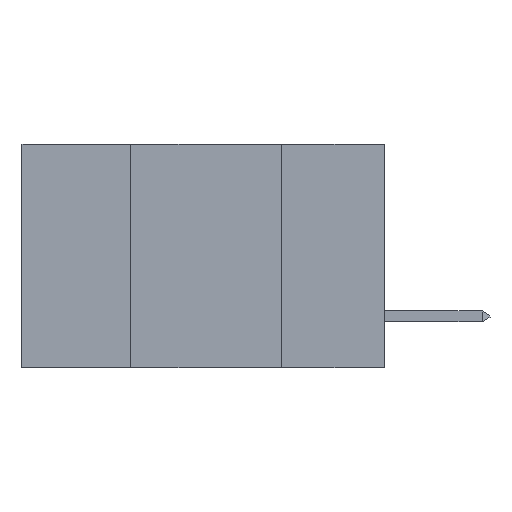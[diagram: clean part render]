
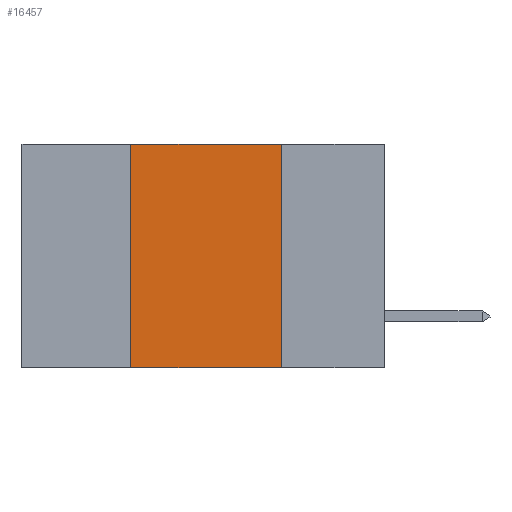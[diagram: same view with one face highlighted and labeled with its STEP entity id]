
A CAD part, left-side view. The second image highlights one B-rep face of the part: STEP entity #16457.
In plain terms, the highlighted planar face has unit normal (-1, 0, 0).
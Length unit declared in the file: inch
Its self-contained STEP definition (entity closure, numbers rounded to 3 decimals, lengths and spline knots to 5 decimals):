
#475 = CARTESIAN_POINT ( 'NONE',  ( 0., 0.17, 0. ) ) ;
#1686 = EDGE_CURVE ( 'NONE', #9627, #5954, #11650, .T. ) ;
#2778 = DIRECTION ( 'NONE',  ( 0., -1., 0. ) ) ;
#2899 = ORIENTED_EDGE ( 'NONE', *, *, #11430, .F. ) ;
#3048 = FACE_OUTER_BOUND ( 'NONE', #17888, .T. ) ;
#3455 = VECTOR ( 'NONE', #4354, 39.37008 ) ;
#3883 = LINE ( 'NONE', #11423, #3455 ) ;
#4007 = DIRECTION ( 'NONE',  ( 1., 0., 0. ) ) ;
#4354 = DIRECTION ( 'NONE',  ( 0., 0., 1. ) ) ;
#4868 = VECTOR ( 'NONE', #18083, 39.37008 ) ;
#5710 = EDGE_CURVE ( 'NONE', #7608, #9627, #11988, .T. ) ;
#5729 = EDGE_CURVE ( 'NONE', #14977, #5954, #8228, .T. ) ;
#5954 = VERTEX_POINT ( 'NONE', #7584 ) ;
#5974 = DIRECTION ( 'NONE',  ( 0., 0., -1. ) ) ;
#6838 = CARTESIAN_POINT ( 'NONE',  ( 0., 0.6, 0. ) ) ;
#7584 = CARTESIAN_POINT ( 'NONE',  ( 0., 0.17, -0.37 ) ) ;
#7608 = VERTEX_POINT ( 'NONE', #12988 ) ;
#7777 = VECTOR ( 'NONE', #2778, 39.37008 ) ;
#7904 = VECTOR ( 'NONE', #5974, 39.37008 ) ;
#8228 = LINE ( 'NONE', #15448, #7777 ) ;
#9627 = VERTEX_POINT ( 'NONE', #475 ) ;
#9691 = PLANE ( 'NONE',  #12712 ) ;
#11423 = CARTESIAN_POINT ( 'NONE',  ( 0., 0.42, 0. ) ) ;
#11430 = EDGE_CURVE ( 'NONE', #14977, #7608, #3883, .T. ) ;
#11650 = LINE ( 'NONE', #12842, #7904 ) ;
#11988 = LINE ( 'NONE', #13955, #4868 ) ;
#12712 = AXIS2_PLACEMENT_3D ( 'NONE', #6838, #4007, #13927 ) ;
#12842 = CARTESIAN_POINT ( 'NONE',  ( 0., 0.17, 0. ) ) ;
#12988 = CARTESIAN_POINT ( 'NONE',  ( 0., 0.42, 0. ) ) ;
#13927 = DIRECTION ( 'NONE',  ( 0., 0., -1. ) ) ;
#13955 = CARTESIAN_POINT ( 'NONE',  ( 0., 0.6, 0. ) ) ;
#14119 = CARTESIAN_POINT ( 'NONE',  ( 0., 0.42, -0.37 ) ) ;
#14303 = ORIENTED_EDGE ( 'NONE', *, *, #1686, .F. ) ;
#14977 = VERTEX_POINT ( 'NONE', #14119 ) ;
#15357 = ORIENTED_EDGE ( 'NONE', *, *, #5710, .F. ) ;
#15448 = CARTESIAN_POINT ( 'NONE',  ( 0., 0.6, -0.37 ) ) ;
#16457 = ADVANCED_FACE ( 'NONE', ( #3048 ), #9691, .F. ) ;
#17861 = ORIENTED_EDGE ( 'NONE', *, *, #5729, .T. ) ;
#17888 = EDGE_LOOP ( 'NONE', ( #14303, #15357, #2899, #17861 ) ) ;
#18083 = DIRECTION ( 'NONE',  ( 0., -1., 0. ) ) ;
